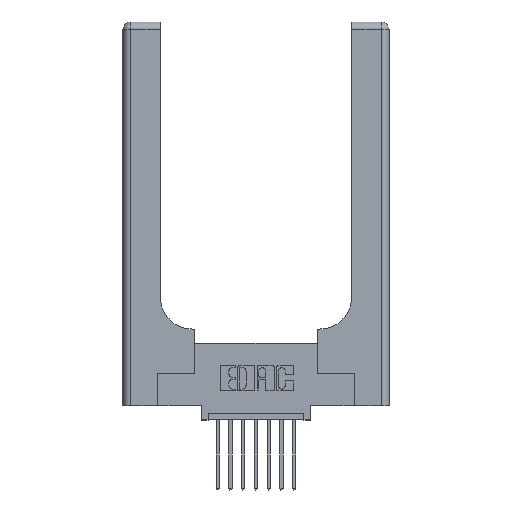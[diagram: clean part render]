
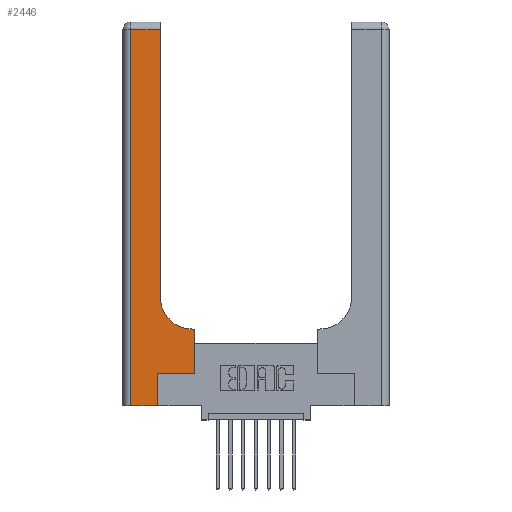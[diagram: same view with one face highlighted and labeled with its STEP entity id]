
A CAD part, top view. The second image highlights one B-rep face of the part: STEP entity #2446.
In plain terms, the highlighted planar face has unit normal (0, 0, 1).
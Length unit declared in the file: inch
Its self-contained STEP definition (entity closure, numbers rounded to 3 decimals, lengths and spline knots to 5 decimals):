
#38 = CARTESIAN_POINT ( 'NONE',  ( 0.2915, 0.6, 0.37 ) ) ;
#640 = EDGE_CURVE ( 'NONE', #2653, #9543, #14486, .T. ) ;
#890 = VECTOR ( 'NONE', #12918, 39.37008 ) ;
#981 = DIRECTION ( 'NONE',  ( 1., 0., 0. ) ) ;
#1076 = CARTESIAN_POINT ( 'NONE',  ( 0., 0., 0.37 ) ) ;
#1270 = ORIENTED_EDGE ( 'NONE', *, *, #13294, .T. ) ;
#1373 = EDGE_CURVE ( 'NONE', #10595, #2653, #3172, .T. ) ;
#1432 = ORIENTED_EDGE ( 'NONE', *, *, #11586, .T. ) ;
#2097 = DIRECTION ( 'NONE',  ( -1., 0., 0. ) ) ;
#2188 = CARTESIAN_POINT ( 'NONE',  ( 0.2915, 0.85, 0.37 ) ) ;
#2194 = VERTEX_POINT ( 'NONE', #14214 ) ;
#2446 = ADVANCED_FACE ( 'NONE', ( #11121 ), #15079, .F. ) ;
#2604 = CARTESIAN_POINT ( 'NONE',  ( 0.269, 0., 0.37 ) ) ;
#2653 = VERTEX_POINT ( 'NONE', #14092 ) ;
#2654 = CARTESIAN_POINT ( 'NONE',  ( 0.5585, 0.6, 0.37 ) ) ;
#2801 = ORIENTED_EDGE ( 'NONE', *, *, #640, .T. ) ;
#2850 = EDGE_CURVE ( 'NONE', #5544, #2194, #5899, .T. ) ;
#3172 = LINE ( 'NONE', #38, #9121 ) ;
#3252 = LINE ( 'NONE', #13206, #4349 ) ;
#3274 = CARTESIAN_POINT ( 'NONE',  ( 0., 3., 0.37 ) ) ;
#3332 = DIRECTION ( 'NONE',  ( 0., -1., 0. ) ) ;
#3454 = DIRECTION ( 'NONE',  ( 0., 0., -1. ) ) ;
#3529 = VERTEX_POINT ( 'NONE', #2604 ) ;
#3842 = LINE ( 'NONE', #1076, #890 ) ;
#4349 = VECTOR ( 'NONE', #8636, 39.37008 ) ;
#4357 = CARTESIAN_POINT ( 'NONE',  ( 0.269, 0.25, 0.37 ) ) ;
#4678 = CARTESIAN_POINT ( 'NONE',  ( 0.06, 3., 0.37 ) ) ;
#4733 = DIRECTION ( 'NONE',  ( 0., 1., 0. ) ) ;
#5083 = LINE ( 'NONE', #4678, #10853 ) ;
#5544 = VERTEX_POINT ( 'NONE', #10919 ) ;
#5672 = DIRECTION ( 'NONE',  ( 1., 0., 0. ) ) ;
#5716 = CARTESIAN_POINT ( 'NONE',  ( 0.269, 0.25, 0.37 ) ) ;
#5847 = EDGE_CURVE ( 'NONE', #9543, #5544, #9490, .T. ) ;
#5899 = LINE ( 'NONE', #13798, #7392 ) ;
#7228 = CARTESIAN_POINT ( 'NONE',  ( 0.2915, 3., 0.37 ) ) ;
#7365 = EDGE_CURVE ( 'NONE', #9728, #3529, #3842, .T. ) ;
#7392 = VECTOR ( 'NONE', #2097, 39.37008 ) ;
#7586 = ORIENTED_EDGE ( 'NONE', *, *, #7365, .T. ) ;
#7885 = VERTEX_POINT ( 'NONE', #14961 ) ;
#7952 = DIRECTION ( 'NONE',  ( -1., 0., 0. ) ) ;
#8278 = EDGE_CURVE ( 'NONE', #7885, #10595, #3252, .T. ) ;
#8636 = DIRECTION ( 'NONE',  ( 0., 1., 0. ) ) ;
#8822 = AXIS2_PLACEMENT_3D ( 'NONE', #12833, #3454, #5672 ) ;
#9121 = VECTOR ( 'NONE', #13581, 39.37008 ) ;
#9413 = CARTESIAN_POINT ( 'NONE',  ( 0.269, 0., 0.37 ) ) ;
#9460 = DIRECTION ( 'NONE',  ( 0., 1., 0. ) ) ;
#9490 = LINE ( 'NONE', #7228, #11125 ) ;
#9543 = VERTEX_POINT ( 'NONE', #2188 ) ;
#9728 = VERTEX_POINT ( 'NONE', #12503 ) ;
#10218 = VECTOR ( 'NONE', #9460, 39.37008 ) ;
#10595 = VERTEX_POINT ( 'NONE', #2654 ) ;
#10853 = VECTOR ( 'NONE', #3332, 39.37008 ) ;
#10919 = CARTESIAN_POINT ( 'NONE',  ( 0.2915, 2.94, 0.37 ) ) ;
#10931 = ORIENTED_EDGE ( 'NONE', *, *, #1373, .T. ) ;
#10944 = VERTEX_POINT ( 'NONE', #4357 ) ;
#11065 = EDGE_CURVE ( 'NONE', #10944, #7885, #12440, .T. ) ;
#11121 = FACE_OUTER_BOUND ( 'NONE', #12512, .T. ) ;
#11125 = VECTOR ( 'NONE', #4733, 39.37008 ) ;
#11459 = DIRECTION ( 'NONE',  ( 0., 0., -1. ) ) ;
#11586 = EDGE_CURVE ( 'NONE', #3529, #10944, #13351, .T. ) ;
#11740 = ORIENTED_EDGE ( 'NONE', *, *, #5847, .T. ) ;
#12081 = ORIENTED_EDGE ( 'NONE', *, *, #11065, .T. ) ;
#12440 = LINE ( 'NONE', #5716, #15220 ) ;
#12503 = CARTESIAN_POINT ( 'NONE',  ( 0.06, 0., 0.37 ) ) ;
#12512 = EDGE_LOOP ( 'NONE', ( #11740, #15203, #1270, #7586, #1432, #12081, #13954, #10931, #2801 ) ) ;
#12766 = AXIS2_PLACEMENT_3D ( 'NONE', #3274, #11459, #7952 ) ;
#12833 = CARTESIAN_POINT ( 'NONE',  ( 0.5415, 0.85, 0.37 ) ) ;
#12918 = DIRECTION ( 'NONE',  ( 1., 0., 0. ) ) ;
#13206 = CARTESIAN_POINT ( 'NONE',  ( 0.5585, 0.25, 0.37 ) ) ;
#13294 = EDGE_CURVE ( 'NONE', #2194, #9728, #5083, .T. ) ;
#13351 = LINE ( 'NONE', #9413, #10218 ) ;
#13581 = DIRECTION ( 'NONE',  ( -1., 0., 0. ) ) ;
#13798 = CARTESIAN_POINT ( 'NONE',  ( 0., 2.94, 0.37 ) ) ;
#13954 = ORIENTED_EDGE ( 'NONE', *, *, #8278, .T. ) ;
#14092 = CARTESIAN_POINT ( 'NONE',  ( 0.5415, 0.6, 0.37 ) ) ;
#14214 = CARTESIAN_POINT ( 'NONE',  ( 0.06, 2.94, 0.37 ) ) ;
#14486 = CIRCLE ( 'NONE', #8822, 0.25 ) ;
#14961 = CARTESIAN_POINT ( 'NONE',  ( 0.5585, 0.25, 0.37 ) ) ;
#15079 = PLANE ( 'NONE',  #12766 ) ;
#15203 = ORIENTED_EDGE ( 'NONE', *, *, #2850, .T. ) ;
#15220 = VECTOR ( 'NONE', #981, 39.37008 ) ;
